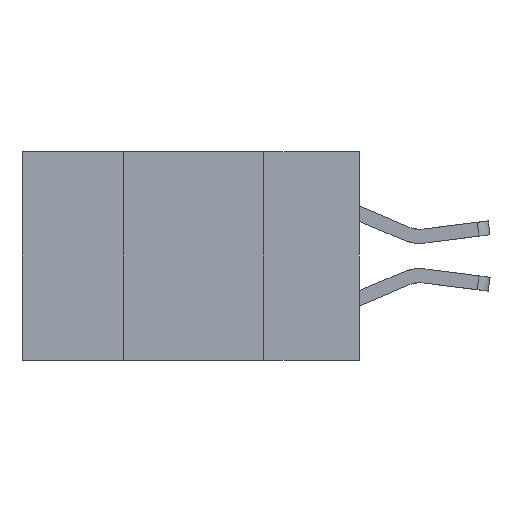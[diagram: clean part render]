
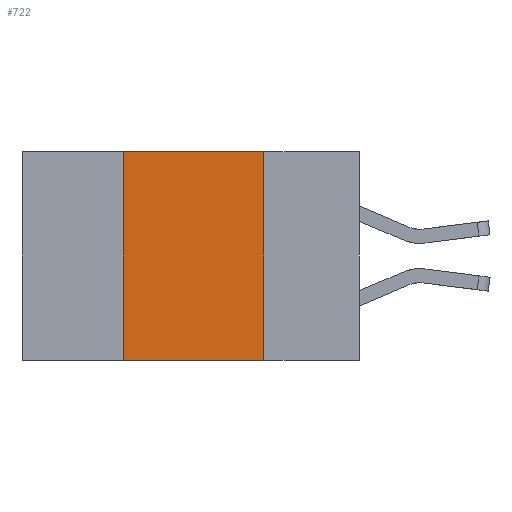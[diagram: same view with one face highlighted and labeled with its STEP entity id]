
A CAD part, left-side view. The second image highlights one B-rep face of the part: STEP entity #722.
In plain terms, the highlighted planar face has unit normal (-1, 0, 0).
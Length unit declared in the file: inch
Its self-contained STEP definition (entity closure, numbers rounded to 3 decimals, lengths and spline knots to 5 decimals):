
#722 = ADVANCED_FACE ( 'NONE', ( #7098 ), #5148, .F. ) ;
#1276 = DIRECTION ( 'NONE',  ( 0., 0., -1. ) ) ;
#1308 = VERTEX_POINT ( 'NONE', #6742 ) ;
#1434 = VERTEX_POINT ( 'NONE', #1985 ) ;
#1498 = EDGE_CURVE ( 'NONE', #1308, #8358, #12000, .T. ) ;
#1659 = ORIENTED_EDGE ( 'NONE', *, *, #3983, .F. ) ;
#1985 = CARTESIAN_POINT ( 'NONE',  ( 0., 0.42, -0.37 ) ) ;
#2232 = AXIS2_PLACEMENT_3D ( 'NONE', #8228, #3261, #1276 ) ;
#2711 = DIRECTION ( 'NONE',  ( 0., 0., 1. ) ) ;
#3261 = DIRECTION ( 'NONE',  ( 1., 0., 0. ) ) ;
#3983 = EDGE_CURVE ( 'NONE', #8358, #6278, #11917, .T. ) ;
#4303 = DIRECTION ( 'NONE',  ( 0., 0., -1. ) ) ;
#4403 = ORIENTED_EDGE ( 'NONE', *, *, #9740, .T. ) ;
#4634 = CARTESIAN_POINT ( 'NONE',  ( 0., 0.42, 0. ) ) ;
#5148 = PLANE ( 'NONE',  #2232 ) ;
#5151 = LINE ( 'NONE', #4634, #6490 ) ;
#5248 = CARTESIAN_POINT ( 'NONE',  ( 0., 0.17, 0. ) ) ;
#5518 = CARTESIAN_POINT ( 'NONE',  ( 0., 0.17, 0. ) ) ;
#5639 = ORIENTED_EDGE ( 'NONE', *, *, #10263, .F. ) ;
#6278 = VERTEX_POINT ( 'NONE', #7882 ) ;
#6366 = ORIENTED_EDGE ( 'NONE', *, *, #1498, .F. ) ;
#6490 = VECTOR ( 'NONE', #2711, 39.37008 ) ;
#6611 = VECTOR ( 'NONE', #9229, 39.37008 ) ;
#6742 = CARTESIAN_POINT ( 'NONE',  ( 0., 0.42, 0. ) ) ;
#7043 = CARTESIAN_POINT ( 'NONE',  ( 0., 0.6, -0.37 ) ) ;
#7098 = FACE_OUTER_BOUND ( 'NONE', #9148, .T. ) ;
#7348 = VECTOR ( 'NONE', #4303, 39.37008 ) ;
#7882 = CARTESIAN_POINT ( 'NONE',  ( 0., 0.17, -0.37 ) ) ;
#8228 = CARTESIAN_POINT ( 'NONE',  ( 0., 0.6, 0. ) ) ;
#8358 = VERTEX_POINT ( 'NONE', #5518 ) ;
#8368 = VECTOR ( 'NONE', #11946, 39.37008 ) ;
#9148 = EDGE_LOOP ( 'NONE', ( #1659, #6366, #5639, #4403 ) ) ;
#9229 = DIRECTION ( 'NONE',  ( 0., -1., 0. ) ) ;
#9740 = EDGE_CURVE ( 'NONE', #1434, #6278, #10334, .T. ) ;
#10263 = EDGE_CURVE ( 'NONE', #1434, #1308, #5151, .T. ) ;
#10334 = LINE ( 'NONE', #7043, #8368 ) ;
#10721 = CARTESIAN_POINT ( 'NONE',  ( 0., 0.6, 0. ) ) ;
#11917 = LINE ( 'NONE', #5248, #7348 ) ;
#11946 = DIRECTION ( 'NONE',  ( 0., -1., 0. ) ) ;
#12000 = LINE ( 'NONE', #10721, #6611 ) ;
